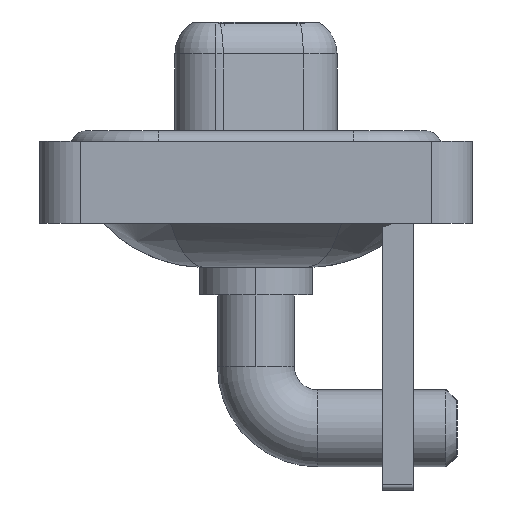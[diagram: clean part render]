
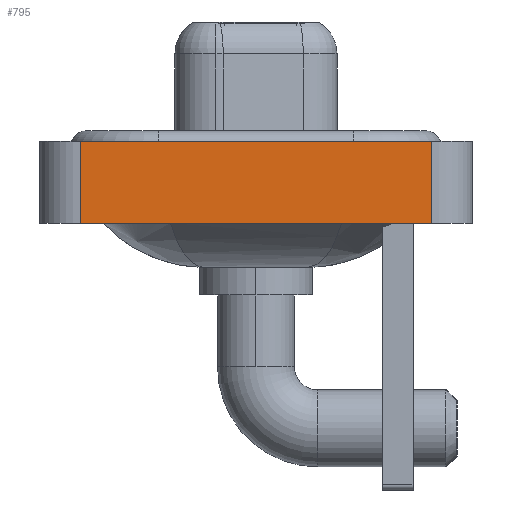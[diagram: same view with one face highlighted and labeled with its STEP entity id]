
A CAD part, left-side view. The second image highlights one B-rep face of the part: STEP entity #795.
In plain terms, the highlighted planar face has unit normal (-1, 0, 0).
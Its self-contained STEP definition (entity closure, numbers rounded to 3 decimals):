
#795 = ADVANCED_FACE ( 'NONE', ( #3841 ), #2732, .T. ) ;
#820 = VERTEX_POINT ( 'NONE', #5487 ) ;
#2260 = ORIENTED_EDGE ( 'NONE', *, *, #4548, .F. ) ;
#2712 = ORIENTED_EDGE ( 'NONE', *, *, #8174, .T. ) ;
#2732 = PLANE ( 'NONE',  #13860 ) ;
#2761 = CARTESIAN_POINT ( 'NONE',  ( -7.3, -8.55, -3.6 ) ) ;
#2873 = CARTESIAN_POINT ( 'NONE',  ( -7.3, 8.55, -3.6 ) ) ;
#3615 = EDGE_CURVE ( 'NONE', #13026, #10954, #14029, .T. ) ;
#3841 = FACE_OUTER_BOUND ( 'NONE', #7630, .T. ) ;
#3928 = CARTESIAN_POINT ( 'NONE',  ( -7.3, -8.55, -3.6 ) ) ;
#4137 = VECTOR ( 'NONE', #9358, 1000. ) ;
#4244 = DIRECTION ( 'NONE',  ( 0., 0., 1. ) ) ;
#4377 = ORIENTED_EDGE ( 'NONE', *, *, #3615, .T. ) ;
#4548 = EDGE_CURVE ( 'NONE', #820, #10954, #4600, .T. ) ;
#4600 = LINE ( 'NONE', #5892, #12261 ) ;
#5487 = CARTESIAN_POINT ( 'NONE',  ( -7.3, 8.55, 0.4 ) ) ;
#5892 = CARTESIAN_POINT ( 'NONE',  ( -7.3, -8.55, 0.4 ) ) ;
#6914 = EDGE_CURVE ( 'NONE', #17921, #820, #17928, .T. ) ;
#7377 = VECTOR ( 'NONE', #9632, 1000. ) ;
#7630 = EDGE_LOOP ( 'NONE', ( #4377, #2260, #16726, #2712 ) ) ;
#7794 = VECTOR ( 'NONE', #4244, 1000. ) ;
#8174 = EDGE_CURVE ( 'NONE', #17921, #13026, #14969, .T. ) ;
#8355 = DIRECTION ( 'NONE',  ( 0., 0., 1. ) ) ;
#9358 = DIRECTION ( 'NONE',  ( 0., -1., 0. ) ) ;
#9632 = DIRECTION ( 'NONE',  ( 0., 0., 1. ) ) ;
#10033 = CARTESIAN_POINT ( 'NONE',  ( -7.3, -8.55, 0.4 ) ) ;
#10747 = CARTESIAN_POINT ( 'NONE',  ( -7.3, -8.55, -3.6 ) ) ;
#10954 = VERTEX_POINT ( 'NONE', #10033 ) ;
#11052 = DIRECTION ( 'NONE',  ( -1., 0., 0. ) ) ;
#11645 = DIRECTION ( 'NONE',  ( 0., -1., 0. ) ) ;
#12261 = VECTOR ( 'NONE', #11645, 1000. ) ;
#13026 = VERTEX_POINT ( 'NONE', #14955 ) ;
#13860 = AXIS2_PLACEMENT_3D ( 'NONE', #3928, #11052, #8355 ) ;
#14029 = LINE ( 'NONE', #2761, #7794 ) ;
#14955 = CARTESIAN_POINT ( 'NONE',  ( -7.3, -8.55, -3.6 ) ) ;
#14969 = LINE ( 'NONE', #10747, #4137 ) ;
#16463 = CARTESIAN_POINT ( 'NONE',  ( -7.3, 8.55, -3.6 ) ) ;
#16726 = ORIENTED_EDGE ( 'NONE', *, *, #6914, .F. ) ;
#17921 = VERTEX_POINT ( 'NONE', #2873 ) ;
#17928 = LINE ( 'NONE', #16463, #7377 ) ;
